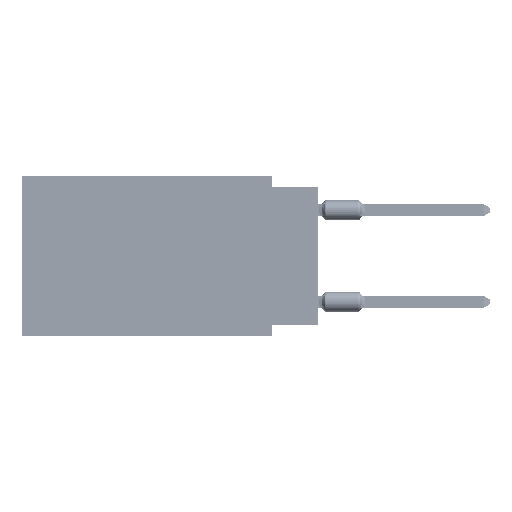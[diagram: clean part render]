
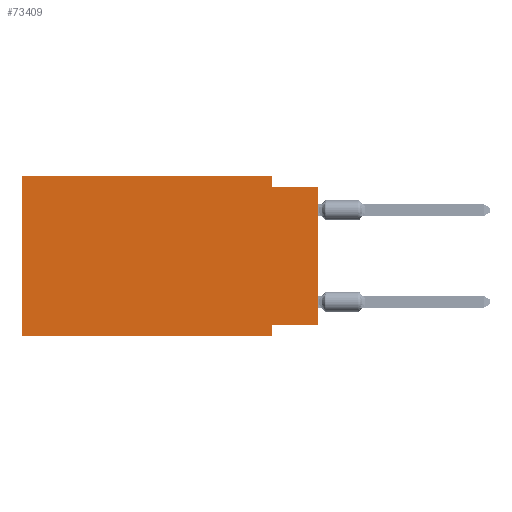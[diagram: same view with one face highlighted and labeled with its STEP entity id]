
A CAD part, left-side view. The second image highlights one B-rep face of the part: STEP entity #73409.
In plain terms, the highlighted planar face has unit normal (-1, 0, 0).
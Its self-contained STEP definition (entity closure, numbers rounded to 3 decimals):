
#165 = DIRECTION ( 'NONE',  ( 1., 0., 0. ) ) ;
#288 = EDGE_CURVE ( 'NONE', #32986, #26002, #31286, .T. ) ;
#1890 = VERTEX_POINT ( 'NONE', #16698 ) ;
#2441 = VERTEX_POINT ( 'NONE', #72463 ) ;
#4013 = EDGE_CURVE ( 'NONE', #1890, #35012, #63156, .T. ) ;
#4360 = DIRECTION ( 'NONE',  ( 0., -1., 0. ) ) ;
#6413 = LINE ( 'NONE', #53730, #28672 ) ;
#10521 = LINE ( 'NONE', #96873, #91417 ) ;
#11322 = VECTOR ( 'NONE', #63161, 1000. ) ;
#12872 = ORIENTED_EDGE ( 'NONE', *, *, #83771, .F. ) ;
#14635 = DIRECTION ( 'NONE',  ( 0., -1., 0. ) ) ;
#15896 = VECTOR ( 'NONE', #56121, 1000. ) ;
#16698 = CARTESIAN_POINT ( 'NONE',  ( 0., 16.383, -8.89 ) ) ;
#24986 = VECTOR ( 'NONE', #86757, 1000. ) ;
#25846 = VECTOR ( 'NONE', #32590, 1000. ) ;
#26002 = VERTEX_POINT ( 'NONE', #65763 ) ;
#27513 = CARTESIAN_POINT ( 'NONE',  ( 0., 2.54, -8.255 ) ) ;
#28672 = VECTOR ( 'NONE', #14635, 1000. ) ;
#31286 = LINE ( 'NONE', #62649, #11322 ) ;
#32590 = DIRECTION ( 'NONE',  ( 0., -1., 0. ) ) ;
#32986 = VERTEX_POINT ( 'NONE', #43154 ) ;
#33095 = CARTESIAN_POINT ( 'NONE',  ( 0., 16.383, 0. ) ) ;
#33968 = EDGE_CURVE ( 'NONE', #35012, #65411, #50032, .T. ) ;
#35012 = VERTEX_POINT ( 'NONE', #98455 ) ;
#40189 = CARTESIAN_POINT ( 'NONE',  ( 0., 2.54, 0. ) ) ;
#41119 = CARTESIAN_POINT ( 'NONE',  ( 0., 2.54, 0. ) ) ;
#42029 = EDGE_CURVE ( 'NONE', #68930, #26002, #59421, .T. ) ;
#42775 = VECTOR ( 'NONE', #97442, 1000. ) ;
#42975 = CARTESIAN_POINT ( 'NONE',  ( 0., 0., -0.635 ) ) ;
#43154 = CARTESIAN_POINT ( 'NONE',  ( 0., 0., -8.255 ) ) ;
#43581 = EDGE_CURVE ( 'NONE', #1890, #2441, #6413, .T. ) ;
#44018 = ORIENTED_EDGE ( 'NONE', *, *, #43581, .T. ) ;
#47197 = CARTESIAN_POINT ( 'NONE',  ( 0., 16.383, 0. ) ) ;
#50032 = LINE ( 'NONE', #33095, #25846 ) ;
#51156 = EDGE_CURVE ( 'NONE', #32986, #71080, #89738, .T. ) ;
#53730 = CARTESIAN_POINT ( 'NONE',  ( 0., 16.383, -8.89 ) ) ;
#56121 = DIRECTION ( 'NONE',  ( 0., 0., -1. ) ) ;
#56573 = ORIENTED_EDGE ( 'NONE', *, *, #288, .T. ) ;
#56662 = AXIS2_PLACEMENT_3D ( 'NONE', #88061, #165, #80353 ) ;
#56816 = DIRECTION ( 'NONE',  ( 0., 0., -1. ) ) ;
#57648 = LINE ( 'NONE', #40189, #15896 ) ;
#58665 = ORIENTED_EDGE ( 'NONE', *, *, #33968, .F. ) ;
#59421 = LINE ( 'NONE', #42975, #100629 ) ;
#62649 = CARTESIAN_POINT ( 'NONE',  ( 0., 0., 0. ) ) ;
#63156 = LINE ( 'NONE', #47197, #24986 ) ;
#63161 = DIRECTION ( 'NONE',  ( 0., 0., 1. ) ) ;
#64453 = PLANE ( 'NONE',  #56662 ) ;
#65411 = VERTEX_POINT ( 'NONE', #41119 ) ;
#65724 = EDGE_CURVE ( 'NONE', #71080, #2441, #10521, .T. ) ;
#65763 = CARTESIAN_POINT ( 'NONE',  ( 0., 0., -0.635 ) ) ;
#67712 = ORIENTED_EDGE ( 'NONE', *, *, #51156, .F. ) ;
#68930 = VERTEX_POINT ( 'NONE', #90055 ) ;
#71080 = VERTEX_POINT ( 'NONE', #27513 ) ;
#72463 = CARTESIAN_POINT ( 'NONE',  ( 0., 2.54, -8.89 ) ) ;
#73409 = ADVANCED_FACE ( 'NONE', ( #94762 ), #64453, .F. ) ;
#80353 = DIRECTION ( 'NONE',  ( 0., 0., -1. ) ) ;
#83771 = EDGE_CURVE ( 'NONE', #65411, #68930, #57648, .T. ) ;
#83780 = ORIENTED_EDGE ( 'NONE', *, *, #4013, .F. ) ;
#86757 = DIRECTION ( 'NONE',  ( 0., 0., 1. ) ) ;
#88061 = CARTESIAN_POINT ( 'NONE',  ( 0., 16.383, 0. ) ) ;
#89229 = CARTESIAN_POINT ( 'NONE',  ( 0., 0., -8.255 ) ) ;
#89738 = LINE ( 'NONE', #89229, #42775 ) ;
#90055 = CARTESIAN_POINT ( 'NONE',  ( 0., 2.54, -0.635 ) ) ;
#91417 = VECTOR ( 'NONE', #56816, 1000. ) ;
#91946 = ORIENTED_EDGE ( 'NONE', *, *, #65724, .F. ) ;
#94762 = FACE_OUTER_BOUND ( 'NONE', #101512, .T. ) ;
#96873 = CARTESIAN_POINT ( 'NONE',  ( 0., 2.54, -8.89 ) ) ;
#97442 = DIRECTION ( 'NONE',  ( 0., 1., 0. ) ) ;
#98455 = CARTESIAN_POINT ( 'NONE',  ( 0., 16.383, 0. ) ) ;
#98494 = ORIENTED_EDGE ( 'NONE', *, *, #42029, .F. ) ;
#100629 = VECTOR ( 'NONE', #4360, 1000. ) ;
#101512 = EDGE_LOOP ( 'NONE', ( #56573, #98494, #12872, #58665, #83780, #44018, #91946, #67712 ) ) ;
